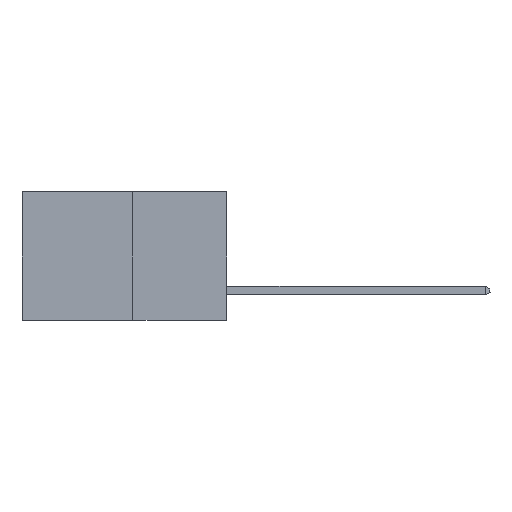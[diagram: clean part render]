
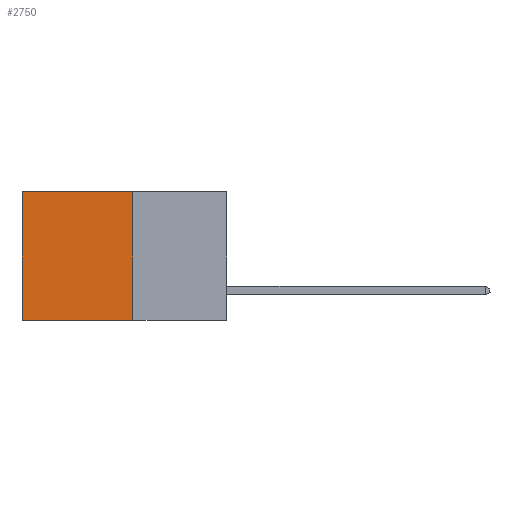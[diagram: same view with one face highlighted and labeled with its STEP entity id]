
A CAD part, left-side view. The second image highlights one B-rep face of the part: STEP entity #2750.
In plain terms, the highlighted planar face has unit normal (-1, 0, 0).
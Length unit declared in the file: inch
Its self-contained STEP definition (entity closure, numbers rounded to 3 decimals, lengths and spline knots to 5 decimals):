
#386 = CARTESIAN_POINT ( 'NONE',  ( 0.277, 0.27, 0. ) ) ;
#787 = VERTEX_POINT ( 'NONE', #386 ) ;
#1233 = EDGE_CURVE ( 'NONE', #787, #6437, #5056, .T. ) ;
#1324 = VECTOR ( 'NONE', #7076, 39.37008 ) ;
#2750 = ADVANCED_FACE ( 'NONE', ( #23294 ), #9977, .F. ) ;
#3414 = CARTESIAN_POINT ( 'NONE',  ( 0.277, 0.27, -0.37 ) ) ;
#5056 = LINE ( 'NONE', #16047, #21411 ) ;
#5114 = EDGE_LOOP ( 'NONE', ( #19411, #20100, #12861, #18818 ) ) ;
#5511 = AXIS2_PLACEMENT_3D ( 'NONE', #9816, #9736, #9691 ) ;
#6178 = LINE ( 'NONE', #3414, #1324 ) ;
#6437 = VERTEX_POINT ( 'NONE', #7441 ) ;
#7076 = DIRECTION ( 'NONE',  ( 0., 1., 0. ) ) ;
#7441 = CARTESIAN_POINT ( 'NONE',  ( 0.277, 0.27, -0.37 ) ) ;
#7932 = VECTOR ( 'NONE', #11554, 39.37008 ) ;
#8006 = DIRECTION ( 'NONE',  ( 0., 0., -1. ) ) ;
#8404 = CARTESIAN_POINT ( 'NONE',  ( 0.277, 0.59, 0. ) ) ;
#8557 = VECTOR ( 'NONE', #20686, 39.37008 ) ;
#9691 = DIRECTION ( 'NONE',  ( 0., 0., -1. ) ) ;
#9736 = DIRECTION ( 'NONE',  ( 1., 0., 0. ) ) ;
#9737 = CARTESIAN_POINT ( 'NONE',  ( 0.277, 0.27, 0. ) ) ;
#9816 = CARTESIAN_POINT ( 'NONE',  ( 0.277, 0.27, -0.37 ) ) ;
#9919 = CARTESIAN_POINT ( 'NONE',  ( 0.277, 0.59, -0.37 ) ) ;
#9977 = PLANE ( 'NONE',  #5511 ) ;
#11554 = DIRECTION ( 'NONE',  ( 0., 1., 0. ) ) ;
#12112 = EDGE_CURVE ( 'NONE', #22181, #12940, #17571, .T. ) ;
#12861 = ORIENTED_EDGE ( 'NONE', *, *, #1233, .F. ) ;
#12940 = VERTEX_POINT ( 'NONE', #19369 ) ;
#15013 = EDGE_CURVE ( 'NONE', #6437, #12940, #6178, .T. ) ;
#16047 = CARTESIAN_POINT ( 'NONE',  ( 0.277, 0.27, -0.37 ) ) ;
#17169 = EDGE_CURVE ( 'NONE', #787, #22181, #22282, .T. ) ;
#17571 = LINE ( 'NONE', #9919, #8557 ) ;
#18818 = ORIENTED_EDGE ( 'NONE', *, *, #17169, .T. ) ;
#19369 = CARTESIAN_POINT ( 'NONE',  ( 0.277, 0.59, -0.37 ) ) ;
#19411 = ORIENTED_EDGE ( 'NONE', *, *, #12112, .T. ) ;
#20100 = ORIENTED_EDGE ( 'NONE', *, *, #15013, .F. ) ;
#20686 = DIRECTION ( 'NONE',  ( 0., 0., -1. ) ) ;
#21411 = VECTOR ( 'NONE', #8006, 39.37008 ) ;
#22181 = VERTEX_POINT ( 'NONE', #8404 ) ;
#22282 = LINE ( 'NONE', #9737, #7932 ) ;
#23294 = FACE_OUTER_BOUND ( 'NONE', #5114, .T. ) ;
